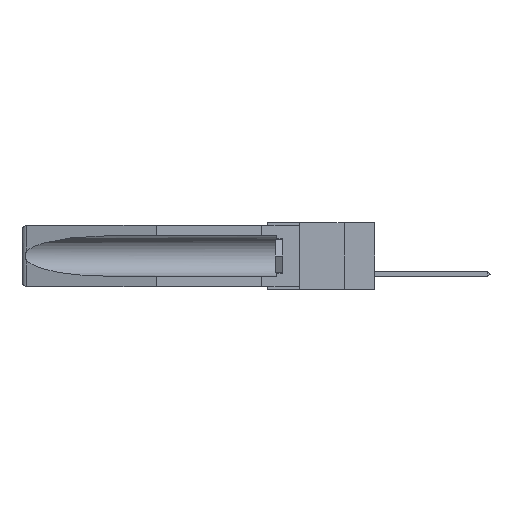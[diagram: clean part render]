
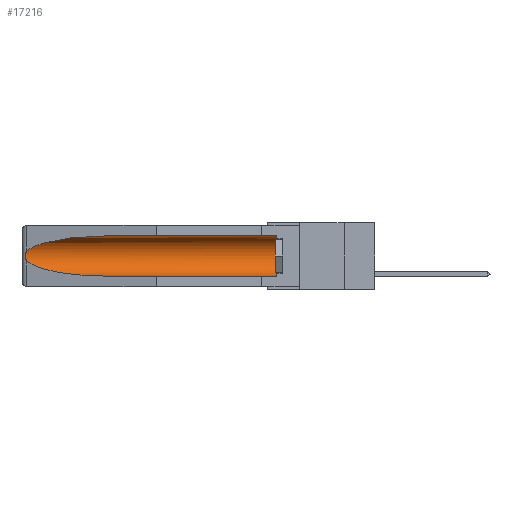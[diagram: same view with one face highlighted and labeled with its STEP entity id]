
A CAD part, left-side view. The second image highlights one B-rep face of the part: STEP entity #17216.
In plain terms, the highlighted cylindrical face has radius 2.857 mm (diameter 5.715 mm), a partial arc.
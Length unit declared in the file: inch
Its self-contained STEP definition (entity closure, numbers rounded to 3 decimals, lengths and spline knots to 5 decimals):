
#222 = CARTESIAN_POINT ( 'NONE',  ( 0.155, -0.30754, -0.059 ) ) ;
#311 = LINE ( 'NONE', #10547, #20114 ) ;
#397 = CARTESIAN_POINT ( 'NONE',  ( 0.26537, 1.52718, -0.14972 ) ) ;
#467 = CARTESIAN_POINT ( 'NONE',  ( 0.2675, 1.53308, -0.17534 ) ) ;
#563 = CARTESIAN_POINT ( 'NONE',  ( 0.155, 1.07973, -0.284 ) ) ;
#789 = CARTESIAN_POINT ( 'NONE',  ( 0.2673, 1.5327, -0.16383 ) ) ;
#880 = AXIS2_PLACEMENT_3D ( 'NONE', #20009, #12815, #21559 ) ;
#1597 = EDGE_CURVE ( 'NONE', #15906, #3243, #9409, .T. ) ;
#2691 = CARTESIAN_POINT ( 'NONE',  ( 0.26597, 1.5296, -0.19026 ) ) ;
#3243 = VERTEX_POINT ( 'NONE', #23374 ) ;
#3426 = EDGE_LOOP ( 'NONE', ( #9297, #20178, #18077, #7101, #17260, #13299 ) ) ;
#3668 = CARTESIAN_POINT ( 'NONE',  ( 0.155, -0.30754, -0.1715 ) ) ;
#4262 = EDGE_CURVE ( 'NONE', #15808, #18960, #9042, .T. ) ;
#4273 = CARTESIAN_POINT ( 'NONE',  ( 0.155, 0.126, -0.059 ) ) ;
#4285 = CARTESIAN_POINT ( 'NONE',  ( 0.26597, 1.52961, -0.15275 ) ) ;
#5714 = CARTESIAN_POINT ( 'NONE',  ( 0.21114, 1.30732, -0.284 ) ) ;
#5783 = CARTESIAN_POINT ( 'NONE',  ( 0.25451, 1.48313, -0.24835 ) ) ;
#6494 = CARTESIAN_POINT ( 'NONE',  ( 0.26537, 1.52718, -0.19328 ) ) ;
#7101 = ORIENTED_EDGE ( 'NONE', *, *, #10611, .F. ) ;
#7901 = CARTESIAN_POINT ( 'NONE',  ( 0.2673, 1.53269, -0.17917 ) ) ;
#7991 = CARTESIAN_POINT ( 'NONE',  ( 0.155, 1.07973, -0.284 ) ) ;
#8296 = VECTOR ( 'NONE', #18729, 39.37008 ) ;
#8529 = EDGE_CURVE ( 'NONE', #3243, #21985, #19124, .T. ) ;
#9039 = DIRECTION ( 'NONE',  ( 0., 1., 0. ) ) ;
#9042 = CIRCLE ( 'NONE', #880, 0.1125 ) ;
#9224 = FACE_OUTER_BOUND ( 'NONE', #3426, .T. ) ;
#9297 = ORIENTED_EDGE ( 'NONE', *, *, #13495, .T. ) ;
#9409 = B_SPLINE_CURVE_WITH_KNOTS ( 'NONE', 3,
 ( #15111, #4285, #16932, #789, #20627, #467, #7901, #9735, #2691, #6494 ),
 .UNSPECIFIED., .F., .F.,
 ( 4, 2, 2, 2, 4 ),
 ( 0., 0.00029, 0.00058, 0.00087, 0.00117 ),
 .UNSPECIFIED. ) ;
#9735 = CARTESIAN_POINT ( 'NONE',  ( 0.26655, 1.53094, -0.18657 ) ) ;
#9739 = CARTESIAN_POINT ( 'NONE',  ( 0.21114, 1.30732, -0.059 ) ) ;
#10547 = CARTESIAN_POINT ( 'NONE',  ( 0.155, -0.30754, -0.284 ) ) ;
#10611 = EDGE_CURVE ( 'NONE', #15808, #21985, #311, .T. ) ;
#11503 = AXIS2_PLACEMENT_3D ( 'NONE', #3668, #9039, #20101 ) ;
#12336 = DIRECTION ( 'NONE',  ( 0., 1., 0. ) ) ;
#12740 = CARTESIAN_POINT ( 'NONE',  ( 0.26537, 1.52718, -0.19328 ) ) ;
#12815 = DIRECTION ( 'NONE',  ( 0., -1., 0. ) ) ;
#13299 = ORIENTED_EDGE ( 'NONE', *, *, #22447, .T. ) ;
#13495 = EDGE_CURVE ( 'NONE', #18737, #15906, #14654, .T. ) ;
#13674 = LINE ( 'NONE', #222, #8296 ) ;
#14654 =( BOUNDED_CURVE ( )  B_SPLINE_CURVE ( 3, ( #15114, #9739, #22010, #397 ),
 .UNSPECIFIED., .F., .T. ) 
 B_SPLINE_CURVE_WITH_KNOTS ( ( 4, 4 ),
 ( 4.71239, 6.08839 ),
 .UNSPECIFIED. ) 
 CURVE ( )  GEOMETRIC_REPRESENTATION_ITEM ( )  RATIONAL_B_SPLINE_CURVE ( ( 1., 0.848, 0.848, 1. ) ) 
 REPRESENTATION_ITEM ( '' )  );
#15111 = CARTESIAN_POINT ( 'NONE',  ( 0.26537, 1.52718, -0.14972 ) ) ;
#15114 = CARTESIAN_POINT ( 'NONE',  ( 0.155, 1.07973, -0.059 ) ) ;
#15747 = CARTESIAN_POINT ( 'NONE',  ( 0.155, 1.07973, -0.059 ) ) ;
#15808 = VERTEX_POINT ( 'NONE', #21138 ) ;
#15906 = VERTEX_POINT ( 'NONE', #20639 ) ;
#16044 = CYLINDRICAL_SURFACE ( 'NONE', #11503, 0.1125 ) ;
#16932 = CARTESIAN_POINT ( 'NONE',  ( 0.26654, 1.53092, -0.15636 ) ) ;
#17216 = ADVANCED_FACE ( 'NONE', ( #9224 ), #16044, .F. ) ;
#17260 = ORIENTED_EDGE ( 'NONE', *, *, #4262, .T. ) ;
#18077 = ORIENTED_EDGE ( 'NONE', *, *, #8529, .T. ) ;
#18729 = DIRECTION ( 'NONE',  ( 0., 1., 0. ) ) ;
#18737 = VERTEX_POINT ( 'NONE', #15747 ) ;
#18960 = VERTEX_POINT ( 'NONE', #4273 ) ;
#19124 =( BOUNDED_CURVE ( )  B_SPLINE_CURVE ( 3, ( #12740, #5783, #5714, #563 ),
 .UNSPECIFIED., .F., .F. ) 
 B_SPLINE_CURVE_WITH_KNOTS ( ( 4, 4 ),
 ( 0.1948, 1.5708 ),
 .UNSPECIFIED. ) 
 CURVE ( )  GEOMETRIC_REPRESENTATION_ITEM ( )  RATIONAL_B_SPLINE_CURVE ( ( 1., 0.848, 0.848, 1. ) ) 
 REPRESENTATION_ITEM ( '' )  );
#20009 = CARTESIAN_POINT ( 'NONE',  ( 0.155, 0.126, -0.1715 ) ) ;
#20101 = DIRECTION ( 'NONE',  ( 0., 0., 1. ) ) ;
#20114 = VECTOR ( 'NONE', #12336, 39.37008 ) ;
#20178 = ORIENTED_EDGE ( 'NONE', *, *, #1597, .T. ) ;
#20627 = CARTESIAN_POINT ( 'NONE',  ( 0.2675, 1.53308, -0.16763 ) ) ;
#20639 = CARTESIAN_POINT ( 'NONE',  ( 0.26537, 1.52718, -0.14972 ) ) ;
#21138 = CARTESIAN_POINT ( 'NONE',  ( 0.155, 0.126, -0.284 ) ) ;
#21559 = DIRECTION ( 'NONE',  ( 0., 0., 1. ) ) ;
#21985 = VERTEX_POINT ( 'NONE', #7991 ) ;
#22010 = CARTESIAN_POINT ( 'NONE',  ( 0.25451, 1.48313, -0.09465 ) ) ;
#22447 = EDGE_CURVE ( 'NONE', #18960, #18737, #13674, .T. ) ;
#23374 = CARTESIAN_POINT ( 'NONE',  ( 0.26537, 1.52718, -0.19328 ) ) ;
